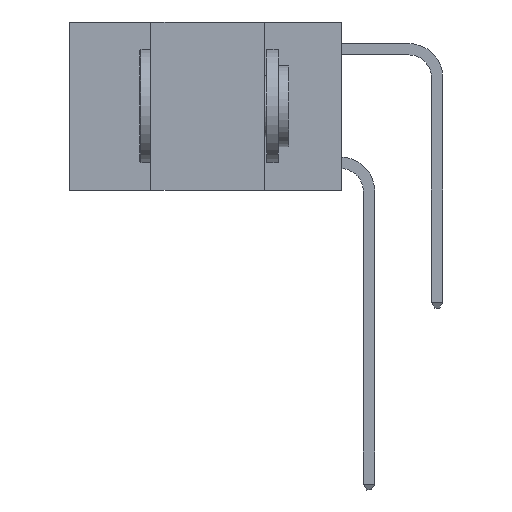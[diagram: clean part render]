
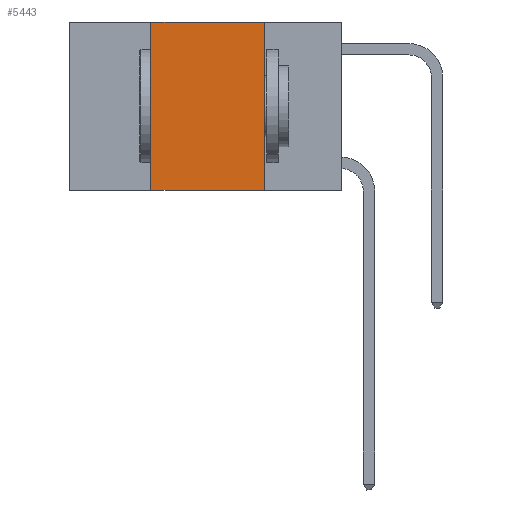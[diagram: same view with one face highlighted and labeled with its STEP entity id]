
A CAD part, left-side view. The second image highlights one B-rep face of the part: STEP entity #5443.
In plain terms, the highlighted planar face has unit normal (-1, 0, 0).
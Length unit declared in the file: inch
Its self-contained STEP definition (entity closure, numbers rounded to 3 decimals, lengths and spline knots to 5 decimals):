
#21 = EDGE_CURVE ( 'NONE', #14400, #11244, #185, .T. ) ;
#185 = LINE ( 'NONE', #8263, #491 ) ;
#309 = DIRECTION ( 'NONE',  ( 0., 0., 1. ) ) ;
#491 = VECTOR ( 'NONE', #1368, 39.37008 ) ;
#641 = VECTOR ( 'NONE', #1170, 39.37008 ) ;
#1170 = DIRECTION ( 'NONE',  ( 0., 0., -1. ) ) ;
#1368 = DIRECTION ( 'NONE',  ( 0., -1., 0. ) ) ;
#1721 = DIRECTION ( 'NONE',  ( 1., 0., 0. ) ) ;
#1827 = EDGE_CURVE ( 'NONE', #11244, #1992, #8060, .T. ) ;
#1855 = ORIENTED_EDGE ( 'NONE', *, *, #21, .F. ) ;
#1992 = VERTEX_POINT ( 'NONE', #13557 ) ;
#2291 = VECTOR ( 'NONE', #6121, 39.37008 ) ;
#2300 = CARTESIAN_POINT ( 'NONE',  ( 0., 0.17, 0. ) ) ;
#2708 = LINE ( 'NONE', #2848, #2291 ) ;
#2848 = CARTESIAN_POINT ( 'NONE',  ( 0., 0.6, -0.37 ) ) ;
#3691 = DIRECTION ( 'NONE',  ( 0., 0., -1. ) ) ;
#4694 = AXIS2_PLACEMENT_3D ( 'NONE', #7199, #1721, #3691 ) ;
#4738 = ORIENTED_EDGE ( 'NONE', *, *, #7529, .F. ) ;
#5443 = ADVANCED_FACE ( 'NONE', ( #11835 ), #6117, .F. ) ;
#5990 = EDGE_CURVE ( 'NONE', #11677, #1992, #2708, .T. ) ;
#6117 = PLANE ( 'NONE',  #4694 ) ;
#6121 = DIRECTION ( 'NONE',  ( 0., -1., 0. ) ) ;
#7199 = CARTESIAN_POINT ( 'NONE',  ( 0., 0.6, 0. ) ) ;
#7281 = LINE ( 'NONE', #8314, #10954 ) ;
#7529 = EDGE_CURVE ( 'NONE', #11677, #14400, #7281, .T. ) ;
#8060 = LINE ( 'NONE', #2300, #641 ) ;
#8068 = EDGE_LOOP ( 'NONE', ( #8629, #1855, #4738, #9344 ) ) ;
#8263 = CARTESIAN_POINT ( 'NONE',  ( 0., 0.6, 0. ) ) ;
#8314 = CARTESIAN_POINT ( 'NONE',  ( 0., 0.42, 0. ) ) ;
#8629 = ORIENTED_EDGE ( 'NONE', *, *, #1827, .F. ) ;
#9344 = ORIENTED_EDGE ( 'NONE', *, *, #5990, .T. ) ;
#10954 = VECTOR ( 'NONE', #309, 39.37008 ) ;
#11244 = VERTEX_POINT ( 'NONE', #13550 ) ;
#11677 = VERTEX_POINT ( 'NONE', #14052 ) ;
#11835 = FACE_OUTER_BOUND ( 'NONE', #8068, .T. ) ;
#12278 = CARTESIAN_POINT ( 'NONE',  ( 0., 0.42, 0. ) ) ;
#13550 = CARTESIAN_POINT ( 'NONE',  ( 0., 0.17, 0. ) ) ;
#13557 = CARTESIAN_POINT ( 'NONE',  ( 0., 0.17, -0.37 ) ) ;
#14052 = CARTESIAN_POINT ( 'NONE',  ( 0., 0.42, -0.37 ) ) ;
#14400 = VERTEX_POINT ( 'NONE', #12278 ) ;
